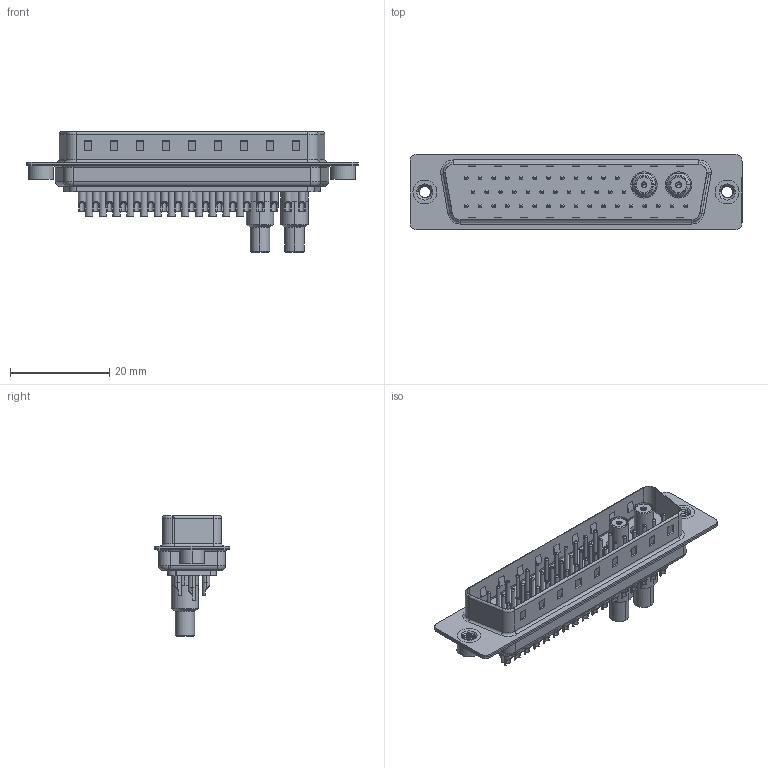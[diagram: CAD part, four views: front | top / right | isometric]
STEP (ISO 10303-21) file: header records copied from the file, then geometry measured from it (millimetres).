
FILE_DESCRIPTION (( 'STEP AP203' ), '1' );
FILE_NAME ('627-43W2622-5NA.STEP', '2019-06-20T02:28:12', ( '' ), ( '' ), 'SwSTEP 2.0', 'SolidWorks 2016', '' );
FILE_SCHEMA (( 'CONFIG_CONTROL_DESIGN' ));
Length unit declared in the file: millimetre
Products named in the file (15): Solder Cover; 627Combo Contact Row 2_22L; 627Combo Shell Rear_50 Contacts; Co-Ax Jack Assy_SC; 627Combo Contact Row 3_22; 627Combo Shell Front_50 Contacts; 627Combo Contact Row 1_22; 627-43W2622-5NA; 627Combo Threaded Rivet_A; Co-Ax Jack_Solder Cup Tail; Insulator Socket; Insulator Socket 2; Locking Collar; Socket_Solder Cup; 627Combo Housing_43W2
Assembly tree (54 placements, depth 3):
  627-43W2622-5NA
    627Combo Housing_43W2
    627Combo Shell Rear_50 Contacts
    627Combo Shell Front_50 Contacts
    627Combo Threaded Rivet_A  x2
    Co-Ax Jack Assy_SC  x2
      Co-Ax Jack_Solder Cup Tail
      Insulator Socket
      Insulator Socket 2
      Locking Collar
      Socket_Solder Cup
      Solder Cover
    627Combo Contact Row 1_22  x12
    627Combo Contact Row 2_22L  x12
    627Combo Contact Row 3_22  x17
Bounding box: 67 x 15.3 x 24.3 mm (x, y, z)
Volume: 4867.1 mm3; surface area: 12788.4 mm2
Topology: 58 solids, 58 shells, 2187 faces, 5073 edges, 3105 vertices
Faces by surface type: cylinder 927, plane 652, torus 468, cone 130, bspline 10
Entity records: 32006 total; most frequent: CARTESIAN_POINT 6696, DIRECTION 5116, ORIENTED_EDGE 4396, EDGE_CURVE 2198, AXIS2_PLACEMENT_3D 2028, VERTEX_POINT 1405, EDGE_LOOP 1183, VECTOR 1060
